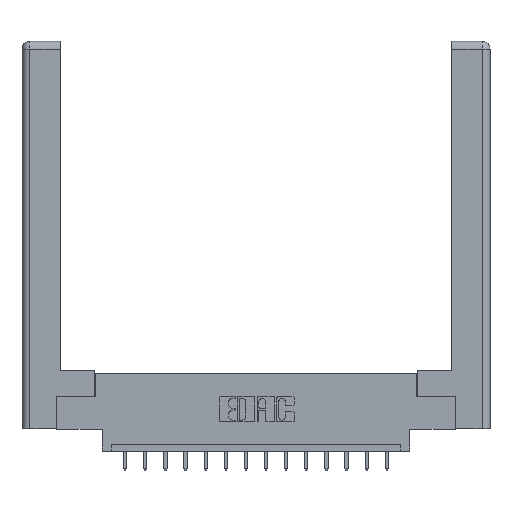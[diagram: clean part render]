
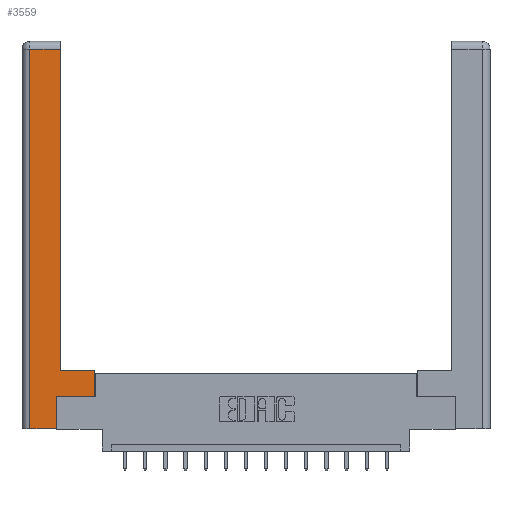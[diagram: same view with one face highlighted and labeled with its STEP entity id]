
A CAD part, top view. The second image highlights one B-rep face of the part: STEP entity #3559.
In plain terms, the highlighted planar face has unit normal (0, 0, 1).
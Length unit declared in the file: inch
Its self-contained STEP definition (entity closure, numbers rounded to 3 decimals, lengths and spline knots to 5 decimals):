
#6 = EDGE_CURVE ( 'NONE', #3486, #2361, #9875, .T. ) ;
#423 = VECTOR ( 'NONE', #3606, 39.37008 ) ;
#617 = DIRECTION ( 'NONE',  ( 1., 0., 0. ) ) ;
#1656 = VERTEX_POINT ( 'NONE', #6970 ) ;
#2122 = LINE ( 'NONE', #4333, #11420 ) ;
#2361 = VERTEX_POINT ( 'NONE', #14594 ) ;
#2439 = VECTOR ( 'NONE', #2658, 39.37008 ) ;
#2548 = CARTESIAN_POINT ( 'NONE',  ( 0.0615, 0., 0. ) ) ;
#2658 = DIRECTION ( 'NONE',  ( -1., 0., 0. ) ) ;
#2663 = DIRECTION ( 'NONE',  ( 0., 1., 0. ) ) ;
#2877 = VERTEX_POINT ( 'NONE', #13053 ) ;
#3140 = EDGE_CURVE ( 'NONE', #8562, #3486, #12881, .T. ) ;
#3486 = VERTEX_POINT ( 'NONE', #12697 ) ;
#3559 = ADVANCED_FACE ( 'NONE', ( #12657 ), #6574, .F. ) ;
#3606 = DIRECTION ( 'NONE',  ( 0., -1., 0. ) ) ;
#4019 = EDGE_CURVE ( 'NONE', #2361, #10525, #12445, .T. ) ;
#4103 = DIRECTION ( 'NONE',  ( -1., 0., 0. ) ) ;
#4333 = CARTESIAN_POINT ( 'NONE',  ( 0.295, 3., 0. ) ) ;
#4966 = EDGE_CURVE ( 'NONE', #14386, #8562, #16490, .T. ) ;
#5010 = AXIS2_PLACEMENT_3D ( 'NONE', #14271, #11703, #4103 ) ;
#5504 = VECTOR ( 'NONE', #12786, 39.37008 ) ;
#5533 = VECTOR ( 'NONE', #2663, 39.37008 ) ;
#5557 = DIRECTION ( 'NONE',  ( 0., 1., 0. ) ) ;
#5760 = CARTESIAN_POINT ( 'NONE',  ( 0.265, 0., 0. ) ) ;
#6257 = LINE ( 'NONE', #15677, #2439 ) ;
#6521 = CARTESIAN_POINT ( 'NONE',  ( 0.565, 0.45, 0. ) ) ;
#6574 = PLANE ( 'NONE',  #5010 ) ;
#6607 = CARTESIAN_POINT ( 'NONE',  ( 0.265, 0.245, 0. ) ) ;
#6742 = DIRECTION ( 'NONE',  ( -1., 0., 0. ) ) ;
#6970 = CARTESIAN_POINT ( 'NONE',  ( 0.295, 2.94, 0. ) ) ;
#7168 = EDGE_CURVE ( 'NONE', #2877, #1656, #2122, .T. ) ;
#7413 = DIRECTION ( 'NONE',  ( 1., 0., 0. ) ) ;
#8310 = VECTOR ( 'NONE', #617, 39.37008 ) ;
#8325 = ORIENTED_EDGE ( 'NONE', *, *, #8818, .T. ) ;
#8562 = VERTEX_POINT ( 'NONE', #5760 ) ;
#8573 = ORIENTED_EDGE ( 'NONE', *, *, #4019, .T. ) ;
#8676 = ORIENTED_EDGE ( 'NONE', *, *, #4966, .T. ) ;
#8818 = EDGE_CURVE ( 'NONE', #10525, #2877, #6257, .T. ) ;
#9875 = LINE ( 'NONE', #12448, #16606 ) ;
#10400 = ORIENTED_EDGE ( 'NONE', *, *, #14789, .T. ) ;
#10525 = VERTEX_POINT ( 'NONE', #6521 ) ;
#11420 = VECTOR ( 'NONE', #5557, 39.37008 ) ;
#11637 = CARTESIAN_POINT ( 'NONE',  ( 0.565, 0.45, 0. ) ) ;
#11703 = DIRECTION ( 'NONE',  ( 0., 0., -1. ) ) ;
#11772 = CARTESIAN_POINT ( 'NONE',  ( 0.0615, 2.94, 0. ) ) ;
#12132 = VERTEX_POINT ( 'NONE', #16200 ) ;
#12411 = ORIENTED_EDGE ( 'NONE', *, *, #3140, .T. ) ;
#12445 = LINE ( 'NONE', #11637, #5504 ) ;
#12448 = CARTESIAN_POINT ( 'NONE',  ( 0.565, 0.245, 0. ) ) ;
#12657 = FACE_OUTER_BOUND ( 'NONE', #13133, .T. ) ;
#12697 = CARTESIAN_POINT ( 'NONE',  ( 0.265, 0.245, 0. ) ) ;
#12786 = DIRECTION ( 'NONE',  ( 0., 1., 0. ) ) ;
#12881 = LINE ( 'NONE', #6607, #5533 ) ;
#12922 = ORIENTED_EDGE ( 'NONE', *, *, #7168, .T. ) ;
#13053 = CARTESIAN_POINT ( 'NONE',  ( 0.295, 0.45, 0. ) ) ;
#13133 = EDGE_LOOP ( 'NONE', ( #12922, #10400, #15463, #8676, #12411, #15875, #8573, #8325 ) ) ;
#13661 = EDGE_CURVE ( 'NONE', #12132, #14386, #15467, .T. ) ;
#14028 = LINE ( 'NONE', #11772, #16495 ) ;
#14271 = CARTESIAN_POINT ( 'NONE',  ( 0., 0., 0. ) ) ;
#14386 = VERTEX_POINT ( 'NONE', #16197 ) ;
#14594 = CARTESIAN_POINT ( 'NONE',  ( 0.565, 0.245, 0. ) ) ;
#14789 = EDGE_CURVE ( 'NONE', #1656, #12132, #14028, .T. ) ;
#15463 = ORIENTED_EDGE ( 'NONE', *, *, #13661, .T. ) ;
#15467 = LINE ( 'NONE', #2548, #423 ) ;
#15677 = CARTESIAN_POINT ( 'NONE',  ( 0.295, 0.45, 0. ) ) ;
#15875 = ORIENTED_EDGE ( 'NONE', *, *, #6, .T. ) ;
#16181 = CARTESIAN_POINT ( 'NONE',  ( 0.265, 0., 0. ) ) ;
#16197 = CARTESIAN_POINT ( 'NONE',  ( 0.0615, 0., 0. ) ) ;
#16200 = CARTESIAN_POINT ( 'NONE',  ( 0.0615, 2.94, 0. ) ) ;
#16490 = LINE ( 'NONE', #16181, #8310 ) ;
#16495 = VECTOR ( 'NONE', #6742, 39.37008 ) ;
#16606 = VECTOR ( 'NONE', #7413, 39.37008 ) ;
